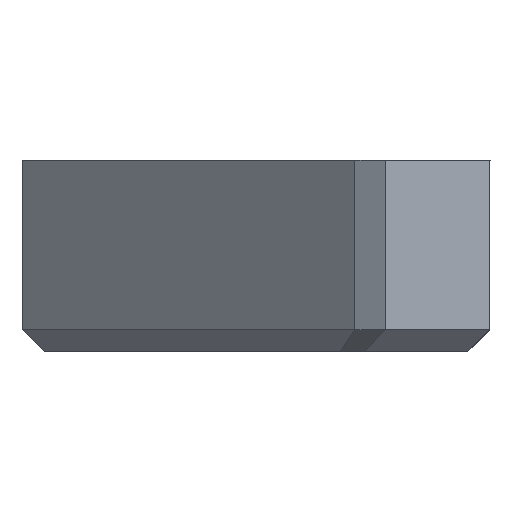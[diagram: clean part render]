
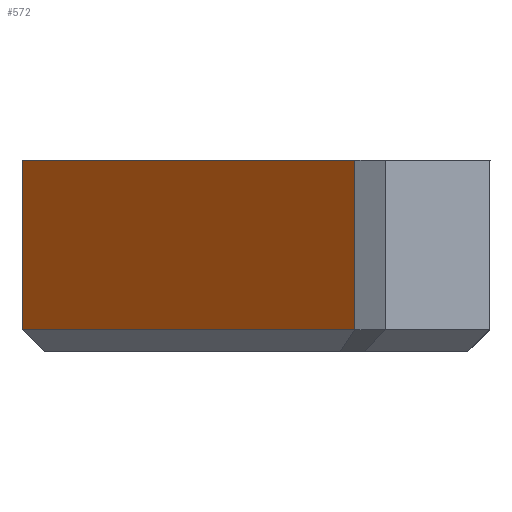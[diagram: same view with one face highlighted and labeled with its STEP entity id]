
A CAD part, left-side view. The second image highlights one B-rep face of the part: STEP entity #572.
In plain terms, the highlighted planar face has unit normal (-0.73, 0.683, 0).
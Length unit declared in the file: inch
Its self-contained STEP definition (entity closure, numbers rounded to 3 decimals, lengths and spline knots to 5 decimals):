
#5 = CARTESIAN_POINT ( 'NONE',  ( -4.91753, 1.3998, 1.21096 ) ) ;
#11 = ORIENTED_EDGE ( 'NONE', *, *, #1401, .F. ) ;
#63 = ORIENTED_EDGE ( 'NONE', *, *, #1339, .T. ) ;
#82 = CARTESIAN_POINT ( 'NONE',  ( -4.47442, 1.873, 3.66447 ) ) ;
#120 = LINE ( 'NONE', #5, #251 ) ;
#174 = CARTESIAN_POINT ( 'NONE',  ( -4.91753, 1.3998, 3.42397 ) ) ;
#209 = CARTESIAN_POINT ( 'NONE',  ( -4.47442, 1.873, 3.42397 ) ) ;
#225 = FACE_OUTER_BOUND ( 'NONE', #1257, .T. ) ;
#245 = VECTOR ( 'NONE', #998, 39.37008 ) ;
#251 = VECTOR ( 'NONE', #1363, 39.37008 ) ;
#297 = VERTEX_POINT ( 'NONE', #420 ) ;
#310 = LINE ( 'NONE', #976, #1098 ) ;
#371 = EDGE_CURVE ( 'NONE', #297, #679, #120, .T. ) ;
#420 = CARTESIAN_POINT ( 'NONE',  ( -4.91753, 1.3998, 3.66447 ) ) ;
#572 = ADVANCED_FACE ( 'NONE', ( #225 ), #1175, .T. ) ;
#589 = LINE ( 'NONE', #1322, #245 ) ;
#669 = ORIENTED_EDGE ( 'NONE', *, *, #371, .F. ) ;
#679 = VERTEX_POINT ( 'NONE', #174 ) ;
#716 = DIRECTION ( 'NONE',  ( -0.73, 0.684, 0. ) ) ;
#838 = DIRECTION ( 'NONE',  ( 0.684, 0.73, 0. ) ) ;
#854 = CARTESIAN_POINT ( 'NONE',  ( -4.47442, 1.873, 2.11446 ) ) ;
#912 = ORIENTED_EDGE ( 'NONE', *, *, #1137, .F. ) ;
#976 = CARTESIAN_POINT ( 'NONE',  ( -4.91753, 1.3998, 3.42397 ) ) ;
#977 = VERTEX_POINT ( 'NONE', #209 ) ;
#998 = DIRECTION ( 'NONE',  ( -0.684, -0.73, 0. ) ) ;
#1023 = LINE ( 'NONE', #854, #1388 ) ;
#1055 = DIRECTION ( 'NONE',  ( 0., 0., 1. ) ) ;
#1098 = VECTOR ( 'NONE', #1313, 39.37008 ) ;
#1137 = EDGE_CURVE ( 'NONE', #977, #1435, #1023, .T. ) ;
#1175 = PLANE ( 'NONE',  #1278 ) ;
#1182 = CARTESIAN_POINT ( 'NONE',  ( -4.92154, 1.39551, 1.21096 ) ) ;
#1257 = EDGE_LOOP ( 'NONE', ( #912, #63, #669, #11 ) ) ;
#1278 = AXIS2_PLACEMENT_3D ( 'NONE', #1182, #716, #838 ) ;
#1313 = DIRECTION ( 'NONE',  ( -0.684, -0.73, 0. ) ) ;
#1322 = CARTESIAN_POINT ( 'NONE',  ( -4.52124, 1.823, 3.66447 ) ) ;
#1339 = EDGE_CURVE ( 'NONE', #977, #679, #310, .T. ) ;
#1363 = DIRECTION ( 'NONE',  ( 0., 0., -1. ) ) ;
#1388 = VECTOR ( 'NONE', #1055, 39.37008 ) ;
#1401 = EDGE_CURVE ( 'NONE', #1435, #297, #589, .T. ) ;
#1435 = VERTEX_POINT ( 'NONE', #82 ) ;
